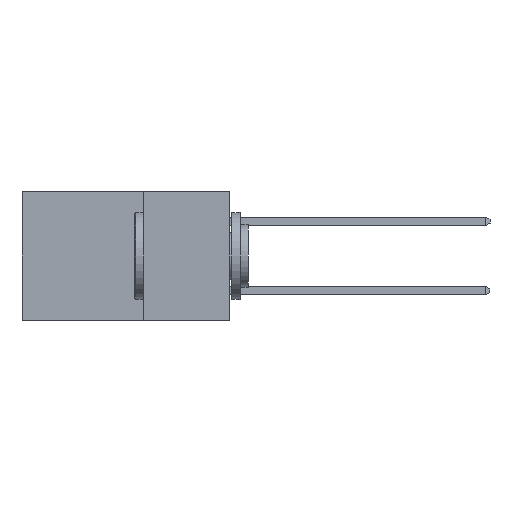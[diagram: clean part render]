
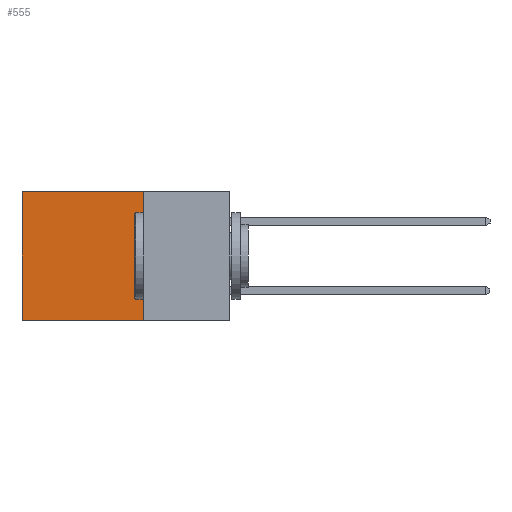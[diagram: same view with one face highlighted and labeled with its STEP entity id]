
A CAD part, left-side view. The second image highlights one B-rep face of the part: STEP entity #555.
In plain terms, the highlighted planar face has unit normal (-1, 0, 0).
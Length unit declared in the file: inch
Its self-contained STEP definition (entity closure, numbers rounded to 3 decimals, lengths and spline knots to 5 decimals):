
#49 = CARTESIAN_POINT ( 'NONE',  ( 0.298, 0.6, 0. ) ) ;
#555 = ADVANCED_FACE ( 'NONE', ( #10022 ), #9519, .F. ) ;
#806 = VECTOR ( 'NONE', #11249, 39.37008 ) ;
#822 = LINE ( 'NONE', #11583, #6872 ) ;
#1674 = EDGE_LOOP ( 'NONE', ( #13772, #15727, #5893, #5163 ) ) ;
#3045 = CARTESIAN_POINT ( 'NONE',  ( 0.298, 0.25, 0. ) ) ;
#3760 = CARTESIAN_POINT ( 'NONE',  ( 0.298, 0.6, -0.37 ) ) ;
#4283 = CARTESIAN_POINT ( 'NONE',  ( 0.298, 0.25, 0. ) ) ;
#5126 = VERTEX_POINT ( 'NONE', #12309 ) ;
#5163 = ORIENTED_EDGE ( 'NONE', *, *, #10654, .T. ) ;
#5631 = AXIS2_PLACEMENT_3D ( 'NONE', #3045, #9284, #12148 ) ;
#5893 = ORIENTED_EDGE ( 'NONE', *, *, #9771, .F. ) ;
#6145 = CARTESIAN_POINT ( 'NONE',  ( 0.298, 0.6, 0. ) ) ;
#6872 = VECTOR ( 'NONE', #12847, 39.37008 ) ;
#7334 = VERTEX_POINT ( 'NONE', #3760 ) ;
#7895 = EDGE_CURVE ( 'NONE', #10459, #7334, #11845, .T. ) ;
#8149 = DIRECTION ( 'NONE',  ( 0., 1., 0. ) ) ;
#9284 = DIRECTION ( 'NONE',  ( 1., 0., 0. ) ) ;
#9419 = VERTEX_POINT ( 'NONE', #15310 ) ;
#9439 = EDGE_CURVE ( 'NONE', #5126, #7334, #822, .T. ) ;
#9519 = PLANE ( 'NONE',  #5631 ) ;
#9771 = EDGE_CURVE ( 'NONE', #9419, #5126, #10999, .T. ) ;
#10017 = CARTESIAN_POINT ( 'NONE',  ( 0.298, 0.25, 0. ) ) ;
#10022 = FACE_OUTER_BOUND ( 'NONE', #1674, .T. ) ;
#10459 = VERTEX_POINT ( 'NONE', #49 ) ;
#10654 = EDGE_CURVE ( 'NONE', #9419, #10459, #14678, .T. ) ;
#10999 = LINE ( 'NONE', #10017, #806 ) ;
#11249 = DIRECTION ( 'NONE',  ( 0., 0., -1. ) ) ;
#11440 = VECTOR ( 'NONE', #12452, 39.37008 ) ;
#11583 = CARTESIAN_POINT ( 'NONE',  ( 0.298, 0.25, -0.37 ) ) ;
#11845 = LINE ( 'NONE', #6145, #11440 ) ;
#12148 = DIRECTION ( 'NONE',  ( 0., 0., -1. ) ) ;
#12309 = CARTESIAN_POINT ( 'NONE',  ( 0.298, 0.25, -0.37 ) ) ;
#12452 = DIRECTION ( 'NONE',  ( 0., 0., -1. ) ) ;
#12847 = DIRECTION ( 'NONE',  ( 0., 1., 0. ) ) ;
#13772 = ORIENTED_EDGE ( 'NONE', *, *, #7895, .T. ) ;
#14303 = VECTOR ( 'NONE', #8149, 39.37008 ) ;
#14678 = LINE ( 'NONE', #4283, #14303 ) ;
#15310 = CARTESIAN_POINT ( 'NONE',  ( 0.298, 0.25, 0. ) ) ;
#15727 = ORIENTED_EDGE ( 'NONE', *, *, #9439, .F. ) ;
